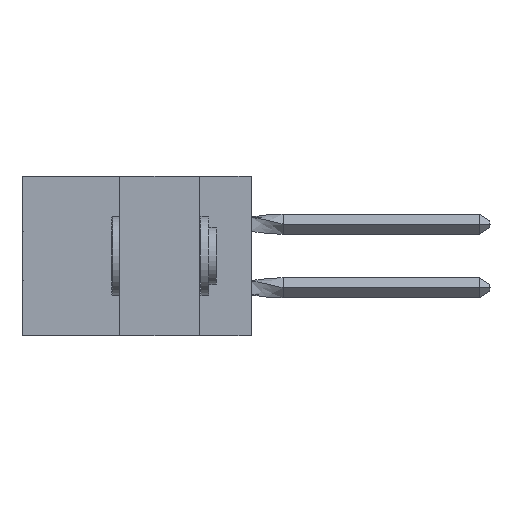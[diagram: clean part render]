
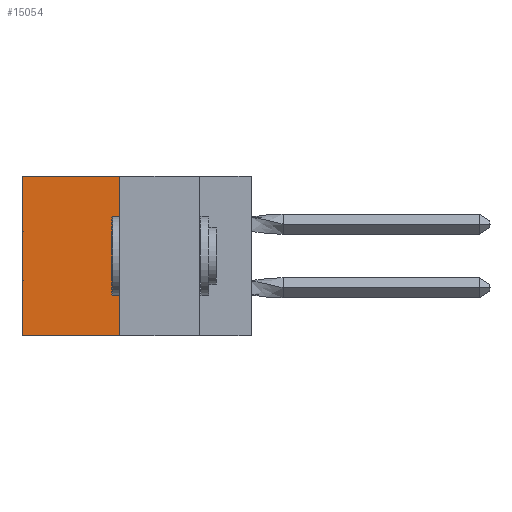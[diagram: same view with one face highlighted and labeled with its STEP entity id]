
A CAD part, left-side view. The second image highlights one B-rep face of the part: STEP entity #15054.
In plain terms, the highlighted planar face has unit normal (-1, 0, 0).
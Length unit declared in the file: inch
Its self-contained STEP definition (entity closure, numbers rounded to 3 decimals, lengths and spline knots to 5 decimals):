
#612 = VERTEX_POINT ( 'NONE', #43305 ) ;
#696 = CARTESIAN_POINT ( 'NONE',  ( 0.305, 0.413, -0.5 ) ) ;
#1018 = LINE ( 'NONE', #7316, #31869 ) ;
#1694 = LINE ( 'NONE', #22377, #15804 ) ;
#3679 = DIRECTION ( 'NONE',  ( 0., 0., -1. ) ) ;
#5400 = ORIENTED_EDGE ( 'NONE', *, *, #34204, .F. ) ;
#5564 = EDGE_LOOP ( 'NONE', ( #34425, #15853, #5400, #33876 ) ) ;
#6791 = EDGE_CURVE ( 'NONE', #39973, #20356, #1694, .T. ) ;
#7316 = CARTESIAN_POINT ( 'NONE',  ( 0.305, 0.72, -0.5 ) ) ;
#7946 = PLANE ( 'NONE',  #39986 ) ;
#12546 = EDGE_CURVE ( 'NONE', #612, #17469, #34469, .T. ) ;
#14386 = DIRECTION ( 'NONE',  ( 0., 0., -1. ) ) ;
#15054 = ADVANCED_FACE ( 'NONE', ( #32662 ), #7946, .F. ) ;
#15090 = CARTESIAN_POINT ( 'NONE',  ( 0.305, 0.413, 0. ) ) ;
#15678 = VECTOR ( 'NONE', #20917, 39.37008 ) ;
#15804 = VECTOR ( 'NONE', #39532, 39.37008 ) ;
#15853 = ORIENTED_EDGE ( 'NONE', *, *, #12546, .F. ) ;
#17469 = VERTEX_POINT ( 'NONE', #20967 ) ;
#20356 = VERTEX_POINT ( 'NONE', #35179 ) ;
#20917 = DIRECTION ( 'NONE',  ( 0., 0., -1. ) ) ;
#20967 = CARTESIAN_POINT ( 'NONE',  ( 0.305, 0.72, -0.5 ) ) ;
#22377 = CARTESIAN_POINT ( 'NONE',  ( 0.305, 0.413, 0. ) ) ;
#24231 = CARTESIAN_POINT ( 'NONE',  ( 0.305, 0.413, -0.5 ) ) ;
#24599 = LINE ( 'NONE', #34517, #15678 ) ;
#28624 = EDGE_CURVE ( 'NONE', #20356, #17469, #1018, .T. ) ;
#31069 = DIRECTION ( 'NONE',  ( 1., 0., 0. ) ) ;
#31869 = VECTOR ( 'NONE', #3679, 39.37008 ) ;
#32662 = FACE_OUTER_BOUND ( 'NONE', #5564, .T. ) ;
#33823 = DIRECTION ( 'NONE',  ( 0., 1., 0. ) ) ;
#33876 = ORIENTED_EDGE ( 'NONE', *, *, #6791, .T. ) ;
#34204 = EDGE_CURVE ( 'NONE', #39973, #612, #24599, .T. ) ;
#34425 = ORIENTED_EDGE ( 'NONE', *, *, #28624, .T. ) ;
#34469 = LINE ( 'NONE', #696, #40735 ) ;
#34517 = CARTESIAN_POINT ( 'NONE',  ( 0.305, 0.413, -0.5 ) ) ;
#35179 = CARTESIAN_POINT ( 'NONE',  ( 0.305, 0.72, 0. ) ) ;
#39532 = DIRECTION ( 'NONE',  ( 0., 1., 0. ) ) ;
#39973 = VERTEX_POINT ( 'NONE', #15090 ) ;
#39986 = AXIS2_PLACEMENT_3D ( 'NONE', #24231, #31069, #14386 ) ;
#40735 = VECTOR ( 'NONE', #33823, 39.37008 ) ;
#43305 = CARTESIAN_POINT ( 'NONE',  ( 0.305, 0.413, -0.5 ) ) ;
